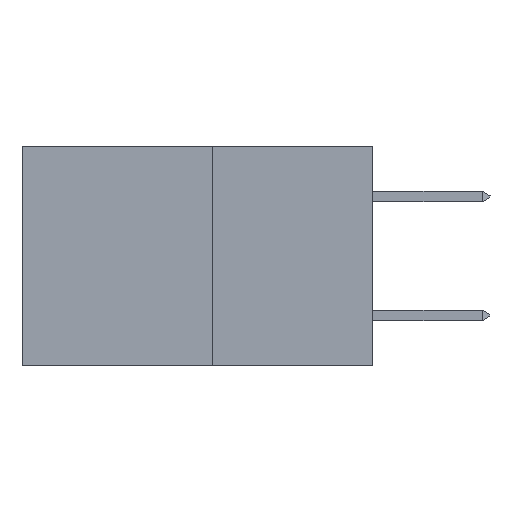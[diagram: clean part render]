
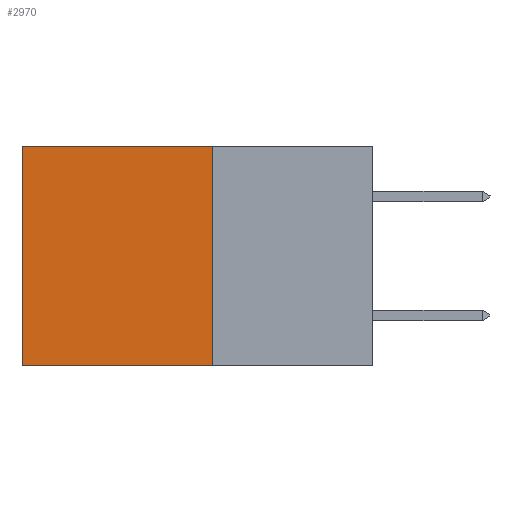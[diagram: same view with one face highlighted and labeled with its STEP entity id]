
A CAD part, left-side view. The second image highlights one B-rep face of the part: STEP entity #2970.
In plain terms, the highlighted planar face has unit normal (-1, 0, 0).
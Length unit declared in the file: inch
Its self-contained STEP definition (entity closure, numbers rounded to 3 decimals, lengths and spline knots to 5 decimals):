
#564 = CARTESIAN_POINT ( 'NONE',  ( 0.277, 0.59, 0. ) ) ;
#971 = FACE_OUTER_BOUND ( 'NONE', #4954, .T. ) ;
#1524 = ORIENTED_EDGE ( 'NONE', *, *, #11524, .T. ) ;
#2040 = AXIS2_PLACEMENT_3D ( 'NONE', #20503, #11179, #12470 ) ;
#2811 = LINE ( 'NONE', #10585, #18630 ) ;
#2970 = ADVANCED_FACE ( 'NONE', ( #971 ), #18251, .F. ) ;
#4176 = CARTESIAN_POINT ( 'NONE',  ( 0.277, 0.59, -0.37 ) ) ;
#4402 = EDGE_CURVE ( 'NONE', #24954, #15334, #9899, .T. ) ;
#4954 = EDGE_LOOP ( 'NONE', ( #1524, #10437, #13169, #22300 ) ) ;
#5090 = VECTOR ( 'NONE', #25591, 39.37008 ) ;
#6289 = DIRECTION ( 'NONE',  ( 0., 0., -1. ) ) ;
#6423 = LINE ( 'NONE', #13350, #5090 ) ;
#6528 = VERTEX_POINT ( 'NONE', #7988 ) ;
#7988 = CARTESIAN_POINT ( 'NONE',  ( 0.277, 0.27, 0. ) ) ;
#9667 = VERTEX_POINT ( 'NONE', #564 ) ;
#9899 = LINE ( 'NONE', #24739, #25601 ) ;
#10437 = ORIENTED_EDGE ( 'NONE', *, *, #4402, .F. ) ;
#10585 = CARTESIAN_POINT ( 'NONE',  ( 0.277, 0.27, 0. ) ) ;
#11179 = DIRECTION ( 'NONE',  ( 1., 0., 0. ) ) ;
#11524 = EDGE_CURVE ( 'NONE', #9667, #15334, #13052, .T. ) ;
#12401 = CARTESIAN_POINT ( 'NONE',  ( 0.277, 0.59, -0.37 ) ) ;
#12470 = DIRECTION ( 'NONE',  ( 0., 0., -1. ) ) ;
#13052 = LINE ( 'NONE', #12401, #17892 ) ;
#13169 = ORIENTED_EDGE ( 'NONE', *, *, #13644, .F. ) ;
#13350 = CARTESIAN_POINT ( 'NONE',  ( 0.277, 0.27, -0.37 ) ) ;
#13644 = EDGE_CURVE ( 'NONE', #6528, #24954, #6423, .T. ) ;
#14678 = EDGE_CURVE ( 'NONE', #6528, #9667, #2811, .T. ) ;
#15334 = VERTEX_POINT ( 'NONE', #4176 ) ;
#16074 = CARTESIAN_POINT ( 'NONE',  ( 0.277, 0.27, -0.37 ) ) ;
#17892 = VECTOR ( 'NONE', #6289, 39.37008 ) ;
#18251 = PLANE ( 'NONE',  #2040 ) ;
#18630 = VECTOR ( 'NONE', #24923, 39.37008 ) ;
#20503 = CARTESIAN_POINT ( 'NONE',  ( 0.277, 0.27, -0.37 ) ) ;
#22300 = ORIENTED_EDGE ( 'NONE', *, *, #14678, .T. ) ;
#24739 = CARTESIAN_POINT ( 'NONE',  ( 0.277, 0.27, -0.37 ) ) ;
#24923 = DIRECTION ( 'NONE',  ( 0., 1., 0. ) ) ;
#24954 = VERTEX_POINT ( 'NONE', #16074 ) ;
#25149 = DIRECTION ( 'NONE',  ( 0., 1., 0. ) ) ;
#25591 = DIRECTION ( 'NONE',  ( 0., 0., -1. ) ) ;
#25601 = VECTOR ( 'NONE', #25149, 39.37008 ) ;
